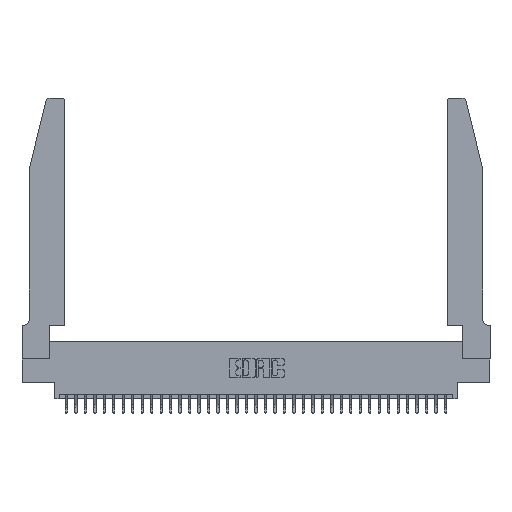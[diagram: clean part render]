
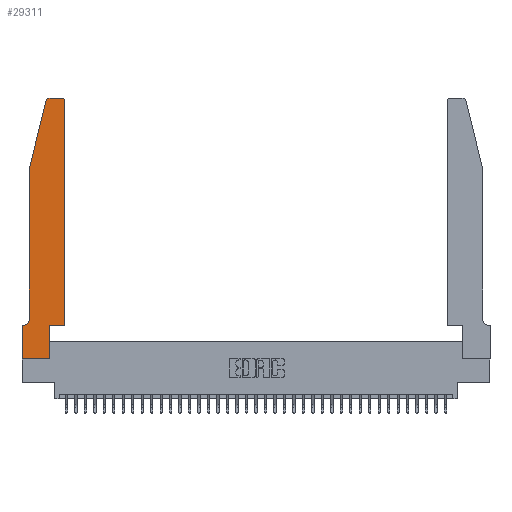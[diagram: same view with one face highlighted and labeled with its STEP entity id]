
A CAD part, top view. The second image highlights one B-rep face of the part: STEP entity #29311.
In plain terms, the highlighted planar face has unit normal (0, 0, 1).
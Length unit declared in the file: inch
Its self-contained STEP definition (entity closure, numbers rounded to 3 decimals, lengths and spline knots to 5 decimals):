
#759 = CARTESIAN_POINT ( 'NONE',  ( 0.4205, 2.75, 0.37 ) ) ;
#837 = DIRECTION ( 'NONE',  ( 0., 1., 0. ) ) ;
#1093 = EDGE_CURVE ( 'NONE', #30752, #20235, #19118, .T. ) ;
#1299 = EDGE_CURVE ( 'NONE', #28187, #2935, #7320, .T. ) ;
#1584 = EDGE_CURVE ( 'NONE', #20235, #23541, #28128, .T. ) ;
#1827 = VERTEX_POINT ( 'NONE', #34855 ) ;
#2020 = AXIS2_PLACEMENT_3D ( 'NONE', #6894, #4210, #36181 ) ;
#2368 = VECTOR ( 'NONE', #36160, 39.37008 ) ;
#2635 = VECTOR ( 'NONE', #837, 39.37008 ) ;
#2935 = VERTEX_POINT ( 'NONE', #759 ) ;
#3873 = VERTEX_POINT ( 'NONE', #19545 ) ;
#4109 = VECTOR ( 'NONE', #23831, 39.37008 ) ;
#4210 = DIRECTION ( 'NONE',  ( 0., 0., 1. ) ) ;
#4824 = VECTOR ( 'NONE', #34464, 39.37008 ) ;
#5121 = LINE ( 'NONE', #35338, #34978 ) ;
#5204 = DIRECTION ( 'NONE',  ( 1., 0., 0. ) ) ;
#5329 = CARTESIAN_POINT ( 'NONE',  ( 0.2865, 0., 0.37 ) ) ;
#5374 = VERTEX_POINT ( 'NONE', #5329 ) ;
#5977 = CARTESIAN_POINT ( 'NONE',  ( 0.0755, 2., 0.37 ) ) ;
#6204 = ORIENTED_EDGE ( 'NONE', *, *, #12481, .T. ) ;
#6423 = CARTESIAN_POINT ( 'NONE',  ( 0.4505, 0.35, 0.37 ) ) ;
#6498 = AXIS2_PLACEMENT_3D ( 'NONE', #25352, #33803, #36937 ) ;
#6702 = EDGE_CURVE ( 'NONE', #5374, #35590, #14897, .T. ) ;
#6894 = CARTESIAN_POINT ( 'NONE',  ( 0.284, 2.72, 0.37 ) ) ;
#7206 = VERTEX_POINT ( 'NONE', #26175 ) ;
#7320 = CIRCLE ( 'NONE', #32227, 0.03 ) ;
#7976 = CIRCLE ( 'NONE', #2020, 0.03 ) ;
#8031 = EDGE_CURVE ( 'NONE', #2935, #3873, #19662, .T. ) ;
#8388 = CARTESIAN_POINT ( 'NONE',  ( 0.4205, 2.72, 0.37 ) ) ;
#8779 = CARTESIAN_POINT ( 'NONE',  ( 0.0755, 2., 0.37 ) ) ;
#8840 = FACE_OUTER_BOUND ( 'NONE', #21229, .T. ) ;
#9200 = ORIENTED_EDGE ( 'NONE', *, *, #28084, .T. ) ;
#9366 = LINE ( 'NONE', #11225, #4824 ) ;
#9564 = AXIS2_PLACEMENT_3D ( 'NONE', #29107, #17836, #17584 ) ;
#10299 = DIRECTION ( 'NONE',  ( 1., 0., 0. ) ) ;
#10340 = VECTOR ( 'NONE', #24992, 39.37008 ) ;
#11170 = CARTESIAN_POINT ( 'NONE',  ( 0.4505, 0.35, 0.37 ) ) ;
#11225 = CARTESIAN_POINT ( 'NONE',  ( 0., 0., 0.37 ) ) ;
#12413 = CIRCLE ( 'NONE', #6498, 0.07 ) ;
#12481 = EDGE_CURVE ( 'NONE', #7206, #1827, #9366, .T. ) ;
#12956 = CARTESIAN_POINT ( 'NONE',  ( 0.4505, 2.72, 0.37 ) ) ;
#13196 = CARTESIAN_POINT ( 'NONE',  ( 0.0755, 2., 0.37 ) ) ;
#13220 = ORIENTED_EDGE ( 'NONE', *, *, #16551, .T. ) ;
#14416 = ORIENTED_EDGE ( 'NONE', *, *, #30123, .T. ) ;
#14897 = LINE ( 'NONE', #32576, #2635 ) ;
#15488 = ORIENTED_EDGE ( 'NONE', *, *, #1093, .T. ) ;
#16551 = EDGE_CURVE ( 'NONE', #17711, #7206, #30158, .T. ) ;
#17254 = ORIENTED_EDGE ( 'NONE', *, *, #1299, .T. ) ;
#17584 = DIRECTION ( 'NONE',  ( 1., 0., 0. ) ) ;
#17711 = VERTEX_POINT ( 'NONE', #35612 ) ;
#17836 = DIRECTION ( 'NONE',  ( 0., 0., 1. ) ) ;
#19118 = LINE ( 'NONE', #13196, #2368 ) ;
#19429 = VECTOR ( 'NONE', #27024, 39.37008 ) ;
#19545 = CARTESIAN_POINT ( 'NONE',  ( 0.284, 2.75, 0.37 ) ) ;
#19662 = LINE ( 'NONE', #24884, #34529 ) ;
#19841 = EDGE_CURVE ( 'NONE', #28479, #28187, #19978, .T. ) ;
#19978 = LINE ( 'NONE', #6423, #19429 ) ;
#20034 = CARTESIAN_POINT ( 'NONE',  ( 0.2865, 0.35, 0.37 ) ) ;
#20076 = EDGE_CURVE ( 'NONE', #23541, #17711, #12413, .T. ) ;
#20235 = VERTEX_POINT ( 'NONE', #8779 ) ;
#20515 = ORIENTED_EDGE ( 'NONE', *, *, #6702, .T. ) ;
#20681 = VECTOR ( 'NONE', #21194, 39.37008 ) ;
#21159 = ORIENTED_EDGE ( 'NONE', *, *, #20076, .T. ) ;
#21194 = DIRECTION ( 'NONE',  ( -1., 0., 0. ) ) ;
#21229 = EDGE_LOOP ( 'NONE', ( #26037, #9200, #15488, #33049, #21159, #13220, #6204, #14416, #20515, #22023, #31097, #17254 ) ) ;
#21926 = CARTESIAN_POINT ( 'NONE',  ( 0.25487, 2.72718, 0.37 ) ) ;
#22023 = ORIENTED_EDGE ( 'NONE', *, *, #32829, .T. ) ;
#23541 = VERTEX_POINT ( 'NONE', #35971 ) ;
#23831 = DIRECTION ( 'NONE',  ( 0., -1., 0. ) ) ;
#24884 = CARTESIAN_POINT ( 'NONE',  ( 0.2605, 2.75, 0.37 ) ) ;
#24992 = DIRECTION ( 'NONE',  ( 1., 0., 0. ) ) ;
#25352 = CARTESIAN_POINT ( 'NONE',  ( 0.0055, 0.42, 0.37 ) ) ;
#26037 = ORIENTED_EDGE ( 'NONE', *, *, #8031, .T. ) ;
#26167 = LINE ( 'NONE', #36695, #10340 ) ;
#26175 = CARTESIAN_POINT ( 'NONE',  ( 0., 0.35, 0.37 ) ) ;
#26888 = DIRECTION ( 'NONE',  ( -1., 0., 0. ) ) ;
#27024 = DIRECTION ( 'NONE',  ( 0., 1., 0. ) ) ;
#27763 = CARTESIAN_POINT ( 'NONE',  ( 0.0755, 0.35, 0.37 ) ) ;
#28084 = EDGE_CURVE ( 'NONE', #3873, #30752, #7976, .T. ) ;
#28128 = LINE ( 'NONE', #5977, #4109 ) ;
#28187 = VERTEX_POINT ( 'NONE', #12956 ) ;
#28479 = VERTEX_POINT ( 'NONE', #11170 ) ;
#29107 = CARTESIAN_POINT ( 'NONE',  ( 0., 0.35, 0.37 ) ) ;
#29311 = ADVANCED_FACE ( 'NONE', ( #8840 ), #34994, .T. ) ;
#30123 = EDGE_CURVE ( 'NONE', #1827, #5374, #5121, .T. ) ;
#30158 = LINE ( 'NONE', #27763, #20681 ) ;
#30752 = VERTEX_POINT ( 'NONE', #21926 ) ;
#31097 = ORIENTED_EDGE ( 'NONE', *, *, #19841, .T. ) ;
#31509 = DIRECTION ( 'NONE',  ( 0., 0., 1. ) ) ;
#32227 = AXIS2_PLACEMENT_3D ( 'NONE', #8388, #31509, #5204 ) ;
#32576 = CARTESIAN_POINT ( 'NONE',  ( 0.2865, 0.35, 0.37 ) ) ;
#32829 = EDGE_CURVE ( 'NONE', #35590, #28479, #26167, .T. ) ;
#33049 = ORIENTED_EDGE ( 'NONE', *, *, #1584, .T. ) ;
#33803 = DIRECTION ( 'NONE',  ( 0., 0., -1. ) ) ;
#34464 = DIRECTION ( 'NONE',  ( 0., -1., 0. ) ) ;
#34529 = VECTOR ( 'NONE', #26888, 39.37008 ) ;
#34855 = CARTESIAN_POINT ( 'NONE',  ( 0., 0., 0.37 ) ) ;
#34978 = VECTOR ( 'NONE', #10299, 39.37008 ) ;
#34994 = PLANE ( 'NONE',  #9564 ) ;
#35338 = CARTESIAN_POINT ( 'NONE',  ( 0., 0., 0.37 ) ) ;
#35590 = VERTEX_POINT ( 'NONE', #20034 ) ;
#35612 = CARTESIAN_POINT ( 'NONE',  ( 0.0055, 0.35, 0.37 ) ) ;
#35971 = CARTESIAN_POINT ( 'NONE',  ( 0.0755, 0.42, 0.37 ) ) ;
#36160 = DIRECTION ( 'NONE',  ( -0.239, -0.971, 0. ) ) ;
#36181 = DIRECTION ( 'NONE',  ( 1., 0., 0. ) ) ;
#36695 = CARTESIAN_POINT ( 'NONE',  ( 0.4505, 0.35, 0.37 ) ) ;
#36937 = DIRECTION ( 'NONE',  ( -1., 0., 0. ) ) ;
